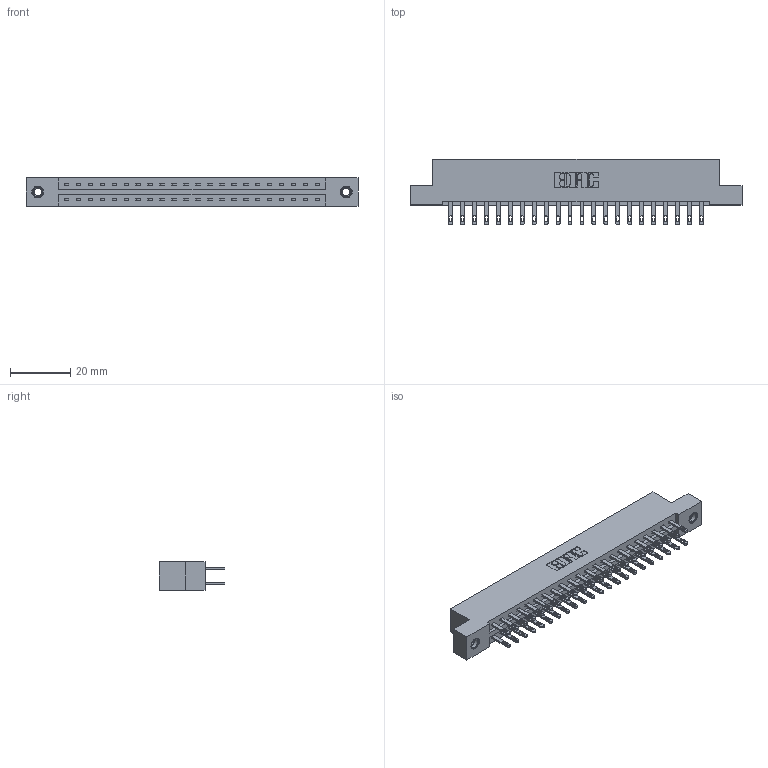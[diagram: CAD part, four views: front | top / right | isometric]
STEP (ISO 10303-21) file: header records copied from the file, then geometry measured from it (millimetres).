
FILE_DESCRIPTION (( 'STEP AP203' ), '1' );
FILE_NAME ('337-044-500-207.STEP', '2019-10-09T12:44:18', ( '' ), ( '' ), 'SwSTEP 2.0', 'SolidWorks 2016', '' );
FILE_SCHEMA (( 'CONFIG_CONTROL_DESIGN' ));
Length unit declared in the file: inch
Products named in the file (4): 337 Part_Flush Mounting Lugs - 0.156 Dia-TI; 337-044-500-207; 345-292-001_345-293-100; 345-250-001_345-250-005-103
Assembly tree (47 placements, depth 2):
  337-044-500-207
    337 Part_Flush Mounting Lugs - 0.156 Dia-TI
    345-292-001_345-293-100  x44
    345-250-001_345-250-005-103  x2
Bounding box: 110.19 x 21.85 x 9.4 mm (x, y, z)
Volume: 11466.9 mm3; surface area: 13293.2 mm2
Topology: 47 solids, 47 shells, 2374 faces, 7179 edges, 4778 vertices
Faces by surface type: plane 1510, cylinder 848, cone 12, torus 4
Entity records: 20760 total; most frequent: CARTESIAN_POINT 3493, ORIENTED_EDGE 3422, DIRECTION 3041, EDGE_CURVE 1711, LINE 1559, VECTOR 1559, VERTEX_POINT 1136, AXIS2_PLACEMENT_3D 741
